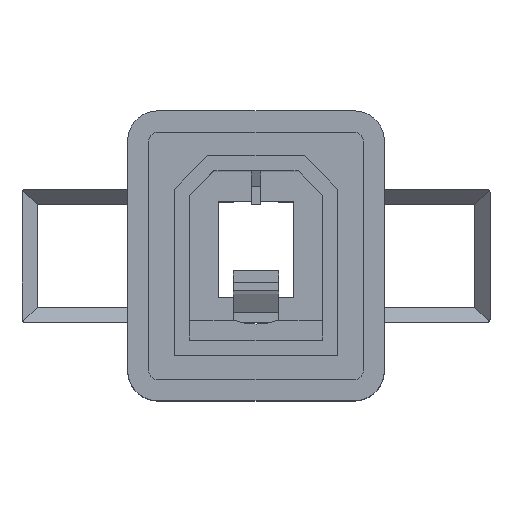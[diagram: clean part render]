
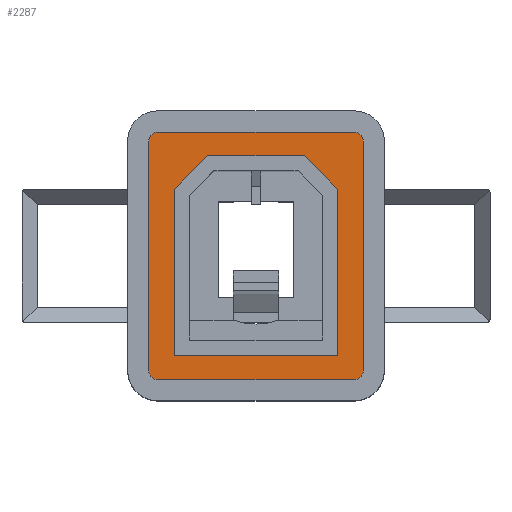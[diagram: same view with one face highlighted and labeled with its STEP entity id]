
A CAD part, top view. The second image highlights one B-rep face of the part: STEP entity #2287.
In plain terms, the highlighted planar face has unit normal (0, 0, 1).
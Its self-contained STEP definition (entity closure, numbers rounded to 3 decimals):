
#27 = LINE ( 'NONE', #3177, #2071 ) ;
#290 = DIRECTION ( 'NONE',  ( 0., -1., 0. ) ) ;
#303 = CIRCLE ( 'NONE', #3279, 0.3 ) ;
#311 = CARTESIAN_POINT ( 'NONE',  ( -3.55, -3.8, 0.5 ) ) ;
#382 = ORIENTED_EDGE ( 'NONE', *, *, #4437, .T. ) ;
#405 = CARTESIAN_POINT ( 'NONE',  ( 1.6, 3.3, 0.5 ) ) ;
#408 = CARTESIAN_POINT ( 'NONE',  ( -3.25, -4.1, 0.5 ) ) ;
#426 = CIRCLE ( 'NONE', #2076, 0.3 ) ;
#487 = CARTESIAN_POINT ( 'NONE',  ( -3.25, 4.1, 0.5 ) ) ;
#601 = VERTEX_POINT ( 'NONE', #3356 ) ;
#619 = VERTEX_POINT ( 'NONE', #1008 ) ;
#702 = VERTEX_POINT ( 'NONE', #4314 ) ;
#744 = ORIENTED_EDGE ( 'NONE', *, *, #1161, .T. ) ;
#746 = VERTEX_POINT ( 'NONE', #3981 ) ;
#814 = VERTEX_POINT ( 'NONE', #408 ) ;
#838 = EDGE_CURVE ( 'NONE', #619, #746, #27, .T. ) ;
#867 = DIRECTION ( 'NONE',  ( 0., 1., 0. ) ) ;
#882 = DIRECTION ( 'NONE',  ( 1., 0., 0. ) ) ;
#896 = EDGE_LOOP ( 'NONE', ( #744, #1726, #2667, #382, #3284, #3622, #3840, #3542 ) ) ;
#942 = DIRECTION ( 'NONE',  ( -1., 0., 0. ) ) ;
#997 = LINE ( 'NONE', #4552, #4346 ) ;
#1008 = CARTESIAN_POINT ( 'NONE',  ( -1.6, 3.3, 0.5 ) ) ;
#1161 = EDGE_CURVE ( 'NONE', #4631, #814, #4446, .T. ) ;
#1183 = CARTESIAN_POINT ( 'NONE',  ( 3.25, -4.1, 0.5 ) ) ;
#1197 = FACE_BOUND ( 'NONE', #2620, .T. ) ;
#1206 = DIRECTION ( 'NONE',  ( -0.707, -0.707, 0. ) ) ;
#1210 = VECTOR ( 'NONE', #2260, 1000. ) ;
#1290 = DIRECTION ( 'NONE',  ( 0., 0., 1. ) ) ;
#1443 = VERTEX_POINT ( 'NONE', #405 ) ;
#1457 = VERTEX_POINT ( 'NONE', #1183 ) ;
#1513 = DIRECTION ( 'NONE',  ( 0., 0., 1. ) ) ;
#1519 = CARTESIAN_POINT ( 'NONE',  ( -2.7, -3.3, 0.5 ) ) ;
#1531 = LINE ( 'NONE', #4964, #4198 ) ;
#1575 = EDGE_CURVE ( 'NONE', #601, #2199, #303, .T. ) ;
#1605 = CARTESIAN_POINT ( 'NONE',  ( 2.7, 2.2, 0.5 ) ) ;
#1608 = CARTESIAN_POINT ( 'NONE',  ( -3.25, -4.1, 0.5 ) ) ;
#1663 = VERTEX_POINT ( 'NONE', #487 ) ;
#1665 = CARTESIAN_POINT ( 'NONE',  ( 3.55, -3.8, 0.5 ) ) ;
#1700 = DIRECTION ( 'NONE',  ( 0., 0., 1. ) ) ;
#1726 = ORIENTED_EDGE ( 'NONE', *, *, #4738, .T. ) ;
#1745 = VECTOR ( 'NONE', #867, 1000. ) ;
#1795 = VECTOR ( 'NONE', #3546, 1000. ) ;
#1895 = DIRECTION ( 'NONE',  ( -1., 0., 0. ) ) ;
#1898 = CARTESIAN_POINT ( 'NONE',  ( -3.25, -3.8, 0.5 ) ) ;
#1967 = LINE ( 'NONE', #1605, #1795 ) ;
#1975 = VECTOR ( 'NONE', #2306, 1000. ) ;
#2066 = EDGE_CURVE ( 'NONE', #4359, #4631, #997, .T. ) ;
#2071 = VECTOR ( 'NONE', #1206, 1000. ) ;
#2076 = AXIS2_PLACEMENT_3D ( 'NONE', #2104, #1290, #942 ) ;
#2080 = EDGE_CURVE ( 'NONE', #2578, #702, #4153, .T. ) ;
#2104 = CARTESIAN_POINT ( 'NONE',  ( 3.25, -3.8, 0.5 ) ) ;
#2199 = VERTEX_POINT ( 'NONE', #3525 ) ;
#2260 = DIRECTION ( 'NONE',  ( 0., 1., 0. ) ) ;
#2271 = DIRECTION ( 'NONE',  ( 0., -1., 0. ) ) ;
#2287 = ADVANCED_FACE ( 'NONE', ( #1197, #2778 ), #4350, .F. ) ;
#2306 = DIRECTION ( 'NONE',  ( -1., 0., 0. ) ) ;
#2314 = ORIENTED_EDGE ( 'NONE', *, *, #2853, .F. ) ;
#2409 = ORIENTED_EDGE ( 'NONE', *, *, #3057, .F. ) ;
#2441 = CARTESIAN_POINT ( 'NONE',  ( -2.7, -3.3, 0.5 ) ) ;
#2447 = EDGE_CURVE ( 'NONE', #2199, #1663, #1531, .T. ) ;
#2485 = AXIS2_PLACEMENT_3D ( 'NONE', #5021, #1513, #3529 ) ;
#2563 = ORIENTED_EDGE ( 'NONE', *, *, #3386, .F. ) ;
#2578 = VERTEX_POINT ( 'NONE', #3498 ) ;
#2591 = CARTESIAN_POINT ( 'NONE',  ( -1.6, 3.3, 0.5 ) ) ;
#2620 = EDGE_LOOP ( 'NONE', ( #2563, #4846, #2693, #2314, #2409, #4170 ) ) ;
#2667 = ORIENTED_EDGE ( 'NONE', *, *, #4336, .T. ) ;
#2693 = ORIENTED_EDGE ( 'NONE', *, *, #838, .F. ) ;
#2778 = FACE_OUTER_BOUND ( 'NONE', #896, .T. ) ;
#2829 = VECTOR ( 'NONE', #2271, 1000. ) ;
#2853 = EDGE_CURVE ( 'NONE', #1443, #619, #4545, .T. ) ;
#3049 = CARTESIAN_POINT ( 'NONE',  ( -2.7, 2.2, 0.5 ) ) ;
#3057 = EDGE_CURVE ( 'NONE', #702, #1443, #1967, .T. ) ;
#3177 = CARTESIAN_POINT ( 'NONE',  ( -2.7, 2.2, 0.5 ) ) ;
#3224 = DIRECTION ( 'NONE',  ( -1., 0., 0. ) ) ;
#3279 = AXIS2_PLACEMENT_3D ( 'NONE', #3667, #1700, #3641 ) ;
#3284 = ORIENTED_EDGE ( 'NONE', *, *, #1575, .T. ) ;
#3295 = AXIS2_PLACEMENT_3D ( 'NONE', #1898, #3603, #3224 ) ;
#3316 = CIRCLE ( 'NONE', #2485, 0.3 ) ;
#3356 = CARTESIAN_POINT ( 'NONE',  ( 3.55, 3.8, 0.5 ) ) ;
#3386 = EDGE_CURVE ( 'NONE', #4345, #2578, #4667, .T. ) ;
#3403 = CARTESIAN_POINT ( 'NONE',  ( 2.7, 2.2, 0.5 ) ) ;
#3479 = DIRECTION ( 'NONE',  ( -1., 0., 0. ) ) ;
#3489 = LINE ( 'NONE', #3049, #2829 ) ;
#3498 = CARTESIAN_POINT ( 'NONE',  ( 2.7, -3.3, 0.5 ) ) ;
#3525 = CARTESIAN_POINT ( 'NONE',  ( 3.25, 4.1, 0.5 ) ) ;
#3529 = DIRECTION ( 'NONE',  ( -1., 0., 0. ) ) ;
#3542 = ORIENTED_EDGE ( 'NONE', *, *, #2066, .T. ) ;
#3546 = DIRECTION ( 'NONE',  ( -0.707, 0.707, 0. ) ) ;
#3564 = DIRECTION ( 'NONE',  ( 1., 0., 0. ) ) ;
#3603 = DIRECTION ( 'NONE',  ( 0., 0., -1. ) ) ;
#3622 = ORIENTED_EDGE ( 'NONE', *, *, #2447, .T. ) ;
#3641 = DIRECTION ( 'NONE',  ( -1., 0., 0. ) ) ;
#3667 = CARTESIAN_POINT ( 'NONE',  ( 3.25, 3.8, 0.5 ) ) ;
#3818 = EDGE_CURVE ( 'NONE', #1663, #4359, #3316, .T. ) ;
#3840 = ORIENTED_EDGE ( 'NONE', *, *, #3818, .T. ) ;
#3895 = DIRECTION ( 'NONE',  ( 0., 0., 1. ) ) ;
#3966 = AXIS2_PLACEMENT_3D ( 'NONE', #4280, #3895, #3479 ) ;
#3981 = CARTESIAN_POINT ( 'NONE',  ( -2.7, 2.2, 0.5 ) ) ;
#3995 = CARTESIAN_POINT ( 'NONE',  ( -3.55, 3.8, 0.5 ) ) ;
#4065 = LINE ( 'NONE', #4419, #1745 ) ;
#4153 = LINE ( 'NONE', #3403, #1210 ) ;
#4170 = ORIENTED_EDGE ( 'NONE', *, *, #2080, .F. ) ;
#4198 = VECTOR ( 'NONE', #1895, 1000. ) ;
#4280 = CARTESIAN_POINT ( 'NONE',  ( -3.25, -3.8, 0.5 ) ) ;
#4293 = VERTEX_POINT ( 'NONE', #1665 ) ;
#4314 = CARTESIAN_POINT ( 'NONE',  ( 2.7, 2.2, 0.5 ) ) ;
#4336 = EDGE_CURVE ( 'NONE', #1457, #4293, #426, .T. ) ;
#4345 = VERTEX_POINT ( 'NONE', #2441 ) ;
#4346 = VECTOR ( 'NONE', #290, 1000. ) ;
#4350 = PLANE ( 'NONE',  #3295 ) ;
#4359 = VERTEX_POINT ( 'NONE', #3995 ) ;
#4419 = CARTESIAN_POINT ( 'NONE',  ( 3.55, -3.8, 0.5 ) ) ;
#4437 = EDGE_CURVE ( 'NONE', #4293, #601, #4065, .T. ) ;
#4446 = CIRCLE ( 'NONE', #3966, 0.3 ) ;
#4463 = VECTOR ( 'NONE', #882, 1000. ) ;
#4545 = LINE ( 'NONE', #2591, #1975 ) ;
#4552 = CARTESIAN_POINT ( 'NONE',  ( -3.55, -3.8, 0.5 ) ) ;
#4631 = VERTEX_POINT ( 'NONE', #311 ) ;
#4667 = LINE ( 'NONE', #1519, #5011 ) ;
#4738 = EDGE_CURVE ( 'NONE', #814, #1457, #4804, .T. ) ;
#4804 = LINE ( 'NONE', #1608, #4463 ) ;
#4846 = ORIENTED_EDGE ( 'NONE', *, *, #5046, .F. ) ;
#4964 = CARTESIAN_POINT ( 'NONE',  ( -3.25, 4.1, 0.5 ) ) ;
#5011 = VECTOR ( 'NONE', #3564, 1000. ) ;
#5021 = CARTESIAN_POINT ( 'NONE',  ( -3.25, 3.8, 0.5 ) ) ;
#5046 = EDGE_CURVE ( 'NONE', #746, #4345, #3489, .T. ) ;
